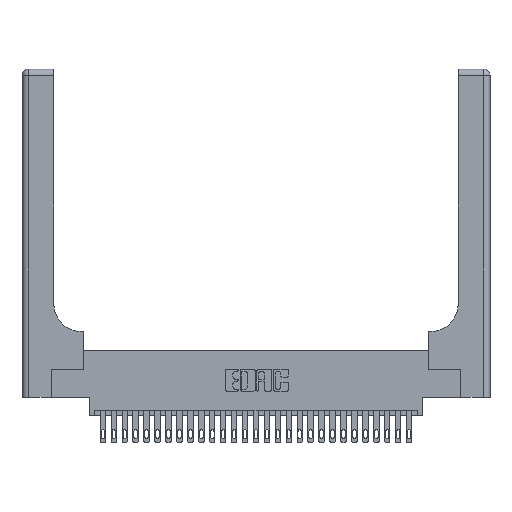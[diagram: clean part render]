
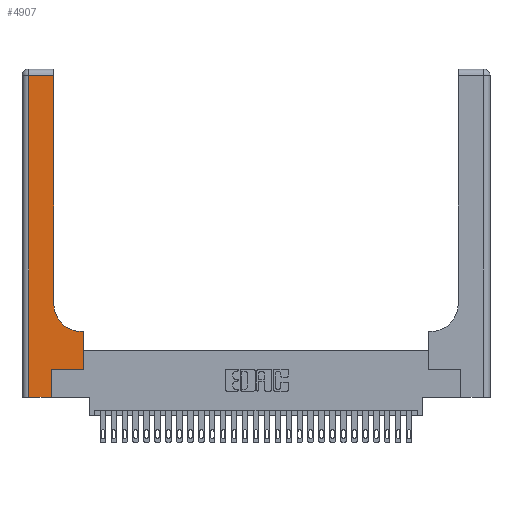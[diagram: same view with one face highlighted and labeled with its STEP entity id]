
A CAD part, top view. The second image highlights one B-rep face of the part: STEP entity #4907.
In plain terms, the highlighted planar face has unit normal (0, 0, 1).
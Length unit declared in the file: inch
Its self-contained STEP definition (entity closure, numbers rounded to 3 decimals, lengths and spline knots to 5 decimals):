
#93 = LINE ( 'NONE', #11254, #19501 ) ;
#161 = ORIENTED_EDGE ( 'NONE', *, *, #26744, .T. ) ;
#207 = LINE ( 'NONE', #2513, #27897 ) ;
#514 = VERTEX_POINT ( 'NONE', #22634 ) ;
#2441 = VERTEX_POINT ( 'NONE', #4781 ) ;
#2513 = CARTESIAN_POINT ( 'NONE',  ( 0., 2.94, 0.37 ) ) ;
#3383 = LINE ( 'NONE', #26505, #14884 ) ;
#3899 = LINE ( 'NONE', #20589, #21506 ) ;
#4419 = VERTEX_POINT ( 'NONE', #24198 ) ;
#4781 = CARTESIAN_POINT ( 'NONE',  ( 0.5585, 0.25, 0.37 ) ) ;
#4907 = ADVANCED_FACE ( 'NONE', ( #9064 ), #21352, .F. ) ;
#6631 = VERTEX_POINT ( 'NONE', #18015 ) ;
#7209 = VECTOR ( 'NONE', #25509, 39.37008 ) ;
#7322 = CARTESIAN_POINT ( 'NONE',  ( 0.269, 0., 0.37 ) ) ;
#7504 = CARTESIAN_POINT ( 'NONE',  ( 0.2915, 2.94, 0.37 ) ) ;
#8189 = EDGE_LOOP ( 'NONE', ( #24482, #161, #25897, #18699, #21019, #28076, #26565, #12742, #17617 ) ) ;
#8269 = EDGE_CURVE ( 'NONE', #4419, #16910, #21113, .T. ) ;
#8877 = CARTESIAN_POINT ( 'NONE',  ( 0.06, 0., 0.37 ) ) ;
#9064 = FACE_OUTER_BOUND ( 'NONE', #8189, .T. ) ;
#9987 = DIRECTION ( 'NONE',  ( 0., 0., -1. ) ) ;
#10188 = DIRECTION ( 'NONE',  ( 1., 0., 0. ) ) ;
#10578 = EDGE_CURVE ( 'NONE', #16910, #514, #93, .T. ) ;
#11254 = CARTESIAN_POINT ( 'NONE',  ( 0., 0., 0.37 ) ) ;
#11352 = DIRECTION ( 'NONE',  ( -1., 0., 0. ) ) ;
#11379 = EDGE_CURVE ( 'NONE', #25925, #24168, #11982, .T. ) ;
#11940 = DIRECTION ( 'NONE',  ( 0., -1., 0. ) ) ;
#11982 = CIRCLE ( 'NONE', #24660, 0.25 ) ;
#12005 = CARTESIAN_POINT ( 'NONE',  ( 0., 3., 0.37 ) ) ;
#12501 = VERTEX_POINT ( 'NONE', #20906 ) ;
#12742 = ORIENTED_EDGE ( 'NONE', *, *, #19486, .T. ) ;
#13269 = EDGE_CURVE ( 'NONE', #514, #12501, #13325, .T. ) ;
#13325 = LINE ( 'NONE', #7322, #7209 ) ;
#14194 = LINE ( 'NONE', #19937, #17389 ) ;
#14326 = DIRECTION ( 'NONE',  ( 0., 0., -1. ) ) ;
#14359 = CARTESIAN_POINT ( 'NONE',  ( 0.06, 3., 0.37 ) ) ;
#14714 = CARTESIAN_POINT ( 'NONE',  ( 0.5415, 0.85, 0.37 ) ) ;
#14884 = VECTOR ( 'NONE', #28715, 39.37008 ) ;
#16910 = VERTEX_POINT ( 'NONE', #8877 ) ;
#17384 = LINE ( 'NONE', #26846, #17737 ) ;
#17389 = VECTOR ( 'NONE', #20291, 39.37008 ) ;
#17617 = ORIENTED_EDGE ( 'NONE', *, *, #11379, .T. ) ;
#17737 = VECTOR ( 'NONE', #22716, 39.37008 ) ;
#17866 = DIRECTION ( 'NONE',  ( 1., 0., 0. ) ) ;
#17975 = VERTEX_POINT ( 'NONE', #7504 ) ;
#18015 = CARTESIAN_POINT ( 'NONE',  ( 0.5585, 0.6, 0.37 ) ) ;
#18699 = ORIENTED_EDGE ( 'NONE', *, *, #10578, .T. ) ;
#19486 = EDGE_CURVE ( 'NONE', #6631, #25925, #3899, .T. ) ;
#19501 = VECTOR ( 'NONE', #17866, 39.37008 ) ;
#19937 = CARTESIAN_POINT ( 'NONE',  ( 0.5585, 0.25, 0.37 ) ) ;
#20291 = DIRECTION ( 'NONE',  ( 0., 1., 0. ) ) ;
#20589 = CARTESIAN_POINT ( 'NONE',  ( 0.2915, 0.6, 0.37 ) ) ;
#20906 = CARTESIAN_POINT ( 'NONE',  ( 0.269, 0.25, 0.37 ) ) ;
#21019 = ORIENTED_EDGE ( 'NONE', *, *, #13269, .T. ) ;
#21113 = LINE ( 'NONE', #14359, #28664 ) ;
#21352 = PLANE ( 'NONE',  #26868 ) ;
#21506 = VECTOR ( 'NONE', #11352, 39.37008 ) ;
#21542 = DIRECTION ( 'NONE',  ( -1., 0., 0. ) ) ;
#21723 = EDGE_CURVE ( 'NONE', #12501, #2441, #17384, .T. ) ;
#22201 = EDGE_CURVE ( 'NONE', #24168, #17975, #3383, .T. ) ;
#22634 = CARTESIAN_POINT ( 'NONE',  ( 0.269, 0., 0.37 ) ) ;
#22716 = DIRECTION ( 'NONE',  ( 1., 0., 0. ) ) ;
#24168 = VERTEX_POINT ( 'NONE', #29508 ) ;
#24198 = CARTESIAN_POINT ( 'NONE',  ( 0.06, 2.94, 0.37 ) ) ;
#24482 = ORIENTED_EDGE ( 'NONE', *, *, #22201, .T. ) ;
#24660 = AXIS2_PLACEMENT_3D ( 'NONE', #14714, #9987, #10188 ) ;
#25509 = DIRECTION ( 'NONE',  ( 0., 1., 0. ) ) ;
#25897 = ORIENTED_EDGE ( 'NONE', *, *, #8269, .T. ) ;
#25925 = VERTEX_POINT ( 'NONE', #29266 ) ;
#26505 = CARTESIAN_POINT ( 'NONE',  ( 0.2915, 3., 0.37 ) ) ;
#26565 = ORIENTED_EDGE ( 'NONE', *, *, #27501, .T. ) ;
#26744 = EDGE_CURVE ( 'NONE', #17975, #4419, #207, .T. ) ;
#26846 = CARTESIAN_POINT ( 'NONE',  ( 0.269, 0.25, 0.37 ) ) ;
#26868 = AXIS2_PLACEMENT_3D ( 'NONE', #12005, #14326, #21542 ) ;
#27501 = EDGE_CURVE ( 'NONE', #2441, #6631, #14194, .T. ) ;
#27897 = VECTOR ( 'NONE', #27928, 39.37008 ) ;
#27928 = DIRECTION ( 'NONE',  ( -1., 0., 0. ) ) ;
#28076 = ORIENTED_EDGE ( 'NONE', *, *, #21723, .T. ) ;
#28664 = VECTOR ( 'NONE', #11940, 39.37008 ) ;
#28715 = DIRECTION ( 'NONE',  ( 0., 1., 0. ) ) ;
#29266 = CARTESIAN_POINT ( 'NONE',  ( 0.5415, 0.6, 0.37 ) ) ;
#29508 = CARTESIAN_POINT ( 'NONE',  ( 0.2915, 0.85, 0.37 ) ) ;
